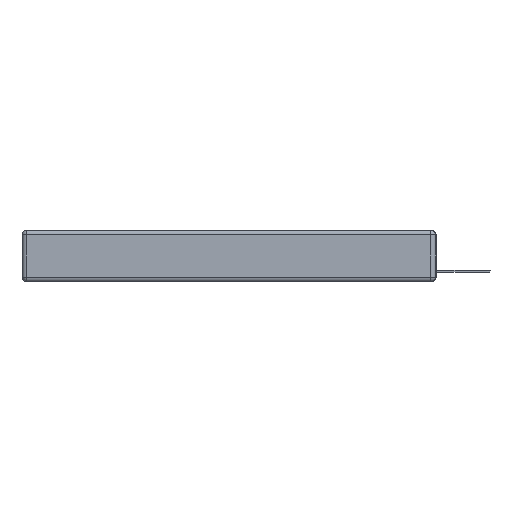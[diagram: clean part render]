
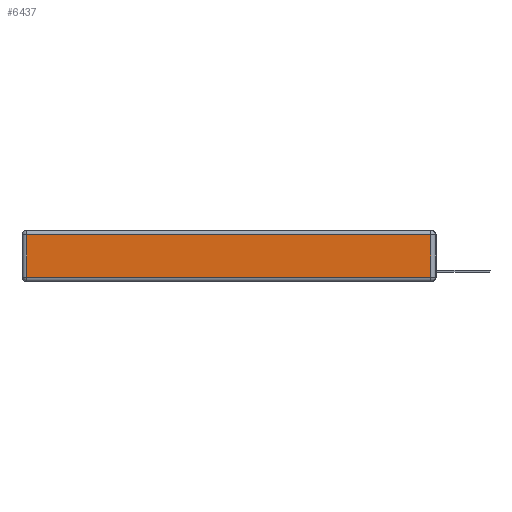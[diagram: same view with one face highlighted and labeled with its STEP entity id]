
A CAD part, left-side view. The second image highlights one B-rep face of the part: STEP entity #6437.
In plain terms, the highlighted planar face has unit normal (-1, 0, 0).
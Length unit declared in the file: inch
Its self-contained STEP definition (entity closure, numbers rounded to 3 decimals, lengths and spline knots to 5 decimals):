
#592 = AXIS2_PLACEMENT_3D ( 'NONE', #1041, #7897, #16541 ) ;
#842 = EDGE_CURVE ( 'NONE', #1328, #21862, #12073, .T. ) ;
#899 = EDGE_CURVE ( 'NONE', #18301, #1328, #7967, .T. ) ;
#932 = VECTOR ( 'NONE', #20285, 39.37008 ) ;
#1041 = CARTESIAN_POINT ( 'NONE',  ( 0., 0., -0.343 ) ) ;
#1328 = VERTEX_POINT ( 'NONE', #16739 ) ;
#2502 = CARTESIAN_POINT ( 'NONE',  ( 0., 0., -0.313 ) ) ;
#3824 = ORIENTED_EDGE ( 'NONE', *, *, #20384, .T. ) ;
#4177 = FACE_OUTER_BOUND ( 'NONE', #9012, .T. ) ;
#4249 = DIRECTION ( 'NONE',  ( 0., -1., 0. ) ) ;
#4821 = CARTESIAN_POINT ( 'NONE',  ( 0., 2.75, -0.03 ) ) ;
#5870 = CARTESIAN_POINT ( 'NONE',  ( 0., 2.72, -0.313 ) ) ;
#6437 = ADVANCED_FACE ( 'NONE', ( #4177 ), #7977, .T. ) ;
#7897 = DIRECTION ( 'NONE',  ( -1., 0., 0. ) ) ;
#7967 = LINE ( 'NONE', #17282, #18079 ) ;
#7977 = PLANE ( 'NONE',  #592 ) ;
#8366 = LINE ( 'NONE', #2502, #12991 ) ;
#9012 = EDGE_LOOP ( 'NONE', ( #3824, #10328, #10080, #11620 ) ) ;
#9093 = VECTOR ( 'NONE', #17209, 39.37008 ) ;
#10080 = ORIENTED_EDGE ( 'NONE', *, *, #842, .T. ) ;
#10328 = ORIENTED_EDGE ( 'NONE', *, *, #899, .T. ) ;
#11593 = EDGE_CURVE ( 'NONE', #21862, #22513, #18968, .T. ) ;
#11620 = ORIENTED_EDGE ( 'NONE', *, *, #11593, .T. ) ;
#12073 = LINE ( 'NONE', #4821, #9093 ) ;
#12991 = VECTOR ( 'NONE', #4249, 39.37008 ) ;
#15754 = DIRECTION ( 'NONE',  ( 0., 0., 1. ) ) ;
#16541 = DIRECTION ( 'NONE',  ( 0., 0., 1. ) ) ;
#16739 = CARTESIAN_POINT ( 'NONE',  ( 0., 0.03, -0.03 ) ) ;
#17209 = DIRECTION ( 'NONE',  ( 0., 1., 0. ) ) ;
#17282 = CARTESIAN_POINT ( 'NONE',  ( 0., 0.03, -0.343 ) ) ;
#17588 = CARTESIAN_POINT ( 'NONE',  ( 0., 2.72, -0.03 ) ) ;
#18079 = VECTOR ( 'NONE', #15754, 39.37008 ) ;
#18301 = VERTEX_POINT ( 'NONE', #19641 ) ;
#18774 = CARTESIAN_POINT ( 'NONE',  ( 0., 2.72, -0.343 ) ) ;
#18968 = LINE ( 'NONE', #18774, #932 ) ;
#19641 = CARTESIAN_POINT ( 'NONE',  ( 0., 0.03, -0.313 ) ) ;
#20285 = DIRECTION ( 'NONE',  ( 0., 0., -1. ) ) ;
#20384 = EDGE_CURVE ( 'NONE', #22513, #18301, #8366, .T. ) ;
#21862 = VERTEX_POINT ( 'NONE', #17588 ) ;
#22513 = VERTEX_POINT ( 'NONE', #5870 ) ;
